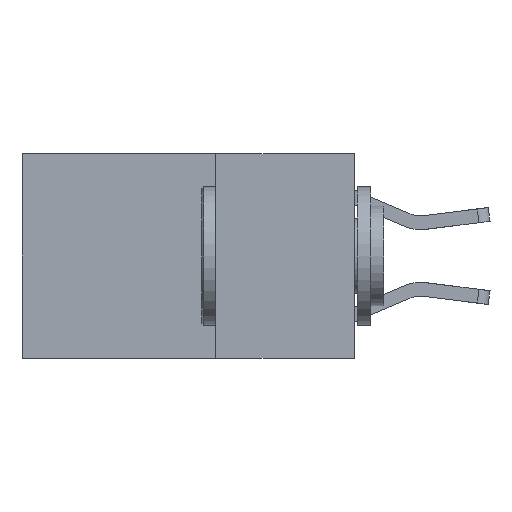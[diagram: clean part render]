
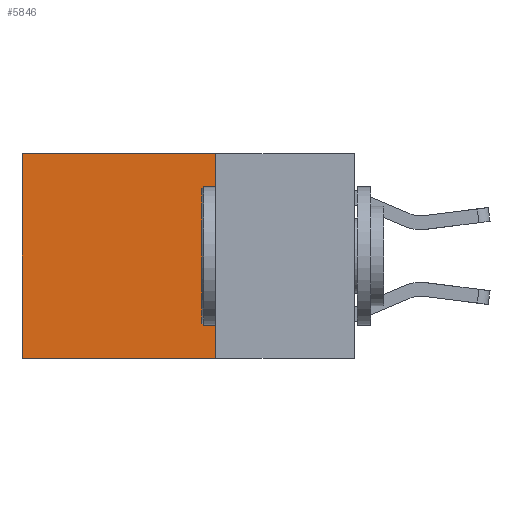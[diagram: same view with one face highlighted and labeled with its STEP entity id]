
A CAD part, left-side view. The second image highlights one B-rep face of the part: STEP entity #5846.
In plain terms, the highlighted planar face has unit normal (-1, 0, 0).
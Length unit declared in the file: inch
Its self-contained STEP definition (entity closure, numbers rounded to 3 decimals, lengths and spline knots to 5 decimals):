
#24 = ORIENTED_EDGE ( 'NONE', *, *, #772, .F. ) ;
#491 = CARTESIAN_POINT ( 'NONE',  ( 0.2625, 0.6, 0. ) ) ;
#772 = EDGE_CURVE ( 'NONE', #2669, #9862, #10103, .T. ) ;
#933 = LINE ( 'NONE', #1135, #9815 ) ;
#1052 = CARTESIAN_POINT ( 'NONE',  ( 0.2625, 0.6, -0.37 ) ) ;
#1116 = AXIS2_PLACEMENT_3D ( 'NONE', #4604, #3894, #3733 ) ;
#1135 = CARTESIAN_POINT ( 'NONE',  ( 0.2625, 0.25, 0. ) ) ;
#1227 = FACE_OUTER_BOUND ( 'NONE', #1290, .T. ) ;
#1290 = EDGE_LOOP ( 'NONE', ( #6892, #4986, #24, #7307 ) ) ;
#1847 = VERTEX_POINT ( 'NONE', #7408 ) ;
#2123 = CARTESIAN_POINT ( 'NONE',  ( 0.2625, 0.25, -0.37 ) ) ;
#2570 = EDGE_CURVE ( 'NONE', #2669, #1847, #933, .T. ) ;
#2669 = VERTEX_POINT ( 'NONE', #8797 ) ;
#2674 = CARTESIAN_POINT ( 'NONE',  ( 0.2625, 0.25, 0. ) ) ;
#2753 = VECTOR ( 'NONE', #8043, 39.37008 ) ;
#3227 = EDGE_CURVE ( 'NONE', #9862, #3522, #8236, .T. ) ;
#3522 = VERTEX_POINT ( 'NONE', #1052 ) ;
#3733 = DIRECTION ( 'NONE',  ( 0., 0., -1. ) ) ;
#3894 = DIRECTION ( 'NONE',  ( 1., 0., 0. ) ) ;
#4452 = DIRECTION ( 'NONE',  ( 0., 1., 0. ) ) ;
#4604 = CARTESIAN_POINT ( 'NONE',  ( 0.2625, 0.25, 0. ) ) ;
#4830 = LINE ( 'NONE', #491, #2753 ) ;
#4986 = ORIENTED_EDGE ( 'NONE', *, *, #3227, .F. ) ;
#5846 = ADVANCED_FACE ( 'NONE', ( #1227 ), #6176, .F. ) ;
#5991 = DIRECTION ( 'NONE',  ( 0., 0., -1. ) ) ;
#6176 = PLANE ( 'NONE',  #1116 ) ;
#6747 = DIRECTION ( 'NONE',  ( 0., 1., 0. ) ) ;
#6892 = ORIENTED_EDGE ( 'NONE', *, *, #10352, .T. ) ;
#7307 = ORIENTED_EDGE ( 'NONE', *, *, #2570, .T. ) ;
#7408 = CARTESIAN_POINT ( 'NONE',  ( 0.2625, 0.6, 0. ) ) ;
#7639 = VECTOR ( 'NONE', #5991, 39.37008 ) ;
#8043 = DIRECTION ( 'NONE',  ( 0., 0., -1. ) ) ;
#8236 = LINE ( 'NONE', #9201, #8289 ) ;
#8289 = VECTOR ( 'NONE', #6747, 39.37008 ) ;
#8797 = CARTESIAN_POINT ( 'NONE',  ( 0.2625, 0.25, 0. ) ) ;
#9201 = CARTESIAN_POINT ( 'NONE',  ( 0.2625, 0.25, -0.37 ) ) ;
#9815 = VECTOR ( 'NONE', #4452, 39.37008 ) ;
#9862 = VERTEX_POINT ( 'NONE', #2123 ) ;
#10103 = LINE ( 'NONE', #2674, #7639 ) ;
#10352 = EDGE_CURVE ( 'NONE', #1847, #3522, #4830, .T. ) ;
